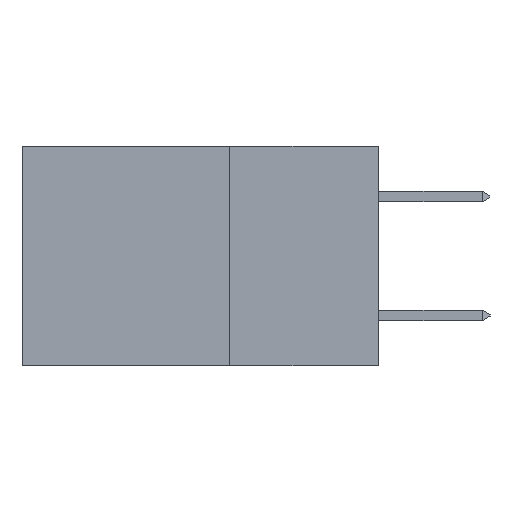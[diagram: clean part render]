
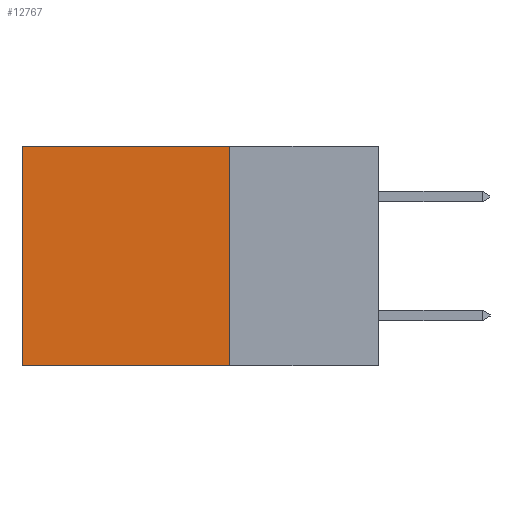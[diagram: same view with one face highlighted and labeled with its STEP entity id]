
A CAD part, left-side view. The second image highlights one B-rep face of the part: STEP entity #12767.
In plain terms, the highlighted planar face has unit normal (-1, 0, 0).
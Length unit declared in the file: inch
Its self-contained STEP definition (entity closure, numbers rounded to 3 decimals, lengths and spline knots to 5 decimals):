
#1678 = ORIENTED_EDGE ( 'NONE', *, *, #7869, .T. ) ;
#1846 = VERTEX_POINT ( 'NONE', #18722 ) ;
#3416 = ORIENTED_EDGE ( 'NONE', *, *, #4695, .T. ) ;
#3584 = CARTESIAN_POINT ( 'NONE',  ( 0.2615, 0.6, -0.37 ) ) ;
#3816 = ORIENTED_EDGE ( 'NONE', *, *, #20266, .F. ) ;
#4695 = EDGE_CURVE ( 'NONE', #1846, #5546, #17686, .T. ) ;
#4753 = FACE_OUTER_BOUND ( 'NONE', #11423, .T. ) ;
#5115 = LINE ( 'NONE', #20907, #22921 ) ;
#5546 = VERTEX_POINT ( 'NONE', #20828 ) ;
#5553 = CARTESIAN_POINT ( 'NONE',  ( 0.2615, 0.25, -0.37 ) ) ;
#5652 = VERTEX_POINT ( 'NONE', #12297 ) ;
#6248 = VECTOR ( 'NONE', #10835, 39.37008 ) ;
#7286 = DIRECTION ( 'NONE',  ( 0., 0., -1. ) ) ;
#7444 = CARTESIAN_POINT ( 'NONE',  ( 0.2615, 0.25, 0. ) ) ;
#7869 = EDGE_CURVE ( 'NONE', #5546, #5652, #20513, .T. ) ;
#8038 = VECTOR ( 'NONE', #21775, 39.37008 ) ;
#8833 = VECTOR ( 'NONE', #18898, 39.37008 ) ;
#10835 = DIRECTION ( 'NONE',  ( 0., 0., -1. ) ) ;
#11174 = EDGE_CURVE ( 'NONE', #11726, #5652, #5115, .T. ) ;
#11423 = EDGE_LOOP ( 'NONE', ( #1678, #14700, #3816, #3416 ) ) ;
#11726 = VERTEX_POINT ( 'NONE', #20811 ) ;
#12075 = DIRECTION ( 'NONE',  ( 0., 1., 0. ) ) ;
#12297 = CARTESIAN_POINT ( 'NONE',  ( 0.2615, 0.6, -0.37 ) ) ;
#12767 = ADVANCED_FACE ( 'NONE', ( #4753 ), #14537, .F. ) ;
#13724 = LINE ( 'NONE', #17133, #8833 ) ;
#14537 = PLANE ( 'NONE',  #21364 ) ;
#14700 = ORIENTED_EDGE ( 'NONE', *, *, #11174, .F. ) ;
#17133 = CARTESIAN_POINT ( 'NONE',  ( 0.2615, 0.25, -0.37 ) ) ;
#17686 = LINE ( 'NONE', #7444, #8038 ) ;
#18123 = DIRECTION ( 'NONE',  ( 1., 0., 0. ) ) ;
#18722 = CARTESIAN_POINT ( 'NONE',  ( 0.2615, 0.25, 0. ) ) ;
#18898 = DIRECTION ( 'NONE',  ( 0., 0., -1. ) ) ;
#20266 = EDGE_CURVE ( 'NONE', #1846, #11726, #13724, .T. ) ;
#20513 = LINE ( 'NONE', #3584, #6248 ) ;
#20811 = CARTESIAN_POINT ( 'NONE',  ( 0.2615, 0.25, -0.37 ) ) ;
#20828 = CARTESIAN_POINT ( 'NONE',  ( 0.2615, 0.6, 0. ) ) ;
#20907 = CARTESIAN_POINT ( 'NONE',  ( 0.2615, 0.25, -0.37 ) ) ;
#21364 = AXIS2_PLACEMENT_3D ( 'NONE', #5553, #18123, #7286 ) ;
#21775 = DIRECTION ( 'NONE',  ( 0., 1., 0. ) ) ;
#22921 = VECTOR ( 'NONE', #12075, 39.37008 ) ;
